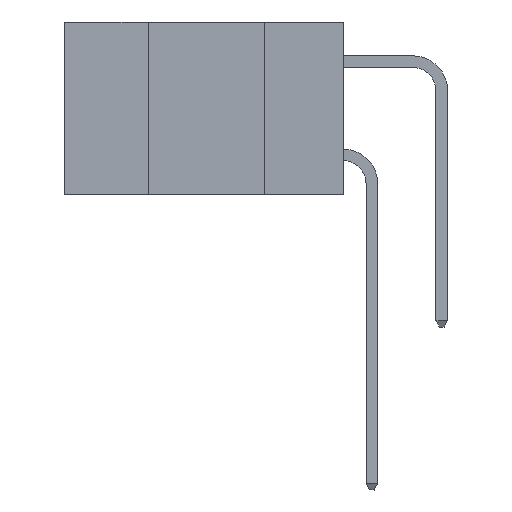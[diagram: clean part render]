
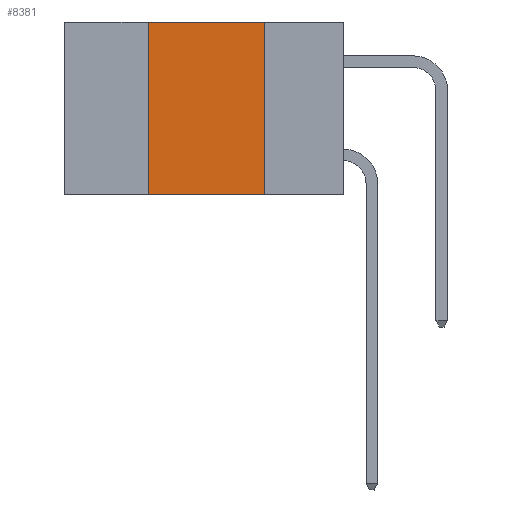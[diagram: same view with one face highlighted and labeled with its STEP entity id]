
A CAD part, left-side view. The second image highlights one B-rep face of the part: STEP entity #8381.
In plain terms, the highlighted planar face has unit normal (-1, 0, 0).
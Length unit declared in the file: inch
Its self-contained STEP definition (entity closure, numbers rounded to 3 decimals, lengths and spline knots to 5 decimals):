
#373 = VERTEX_POINT ( 'NONE', #10980 ) ;
#387 = LINE ( 'NONE', #440, #10869 ) ;
#440 = CARTESIAN_POINT ( 'NONE',  ( 0., 0.6, -0.37 ) ) ;
#542 = CARTESIAN_POINT ( 'NONE',  ( 0., 0.42, -0.37 ) ) ;
#835 = CARTESIAN_POINT ( 'NONE',  ( 0., 0.6, 0. ) ) ;
#958 = ORIENTED_EDGE ( 'NONE', *, *, #9473, .F. ) ;
#2088 = EDGE_CURVE ( 'NONE', #373, #5989, #387, .T. ) ;
#2133 = ORIENTED_EDGE ( 'NONE', *, *, #7985, .F. ) ;
#2447 = EDGE_CURVE ( 'NONE', #2599, #5989, #9921, .T. ) ;
#2492 = VECTOR ( 'NONE', #5140, 39.37008 ) ;
#2599 = VERTEX_POINT ( 'NONE', #11476 ) ;
#3918 = DIRECTION ( 'NONE',  ( 0., 0., -1. ) ) ;
#3961 = LINE ( 'NONE', #9035, #8704 ) ;
#5140 = DIRECTION ( 'NONE',  ( 0., 0., 1. ) ) ;
#5313 = VECTOR ( 'NONE', #3918, 39.37008 ) ;
#5989 = VERTEX_POINT ( 'NONE', #7119 ) ;
#6119 = FACE_OUTER_BOUND ( 'NONE', #9298, .T. ) ;
#7119 = CARTESIAN_POINT ( 'NONE',  ( 0., 0.17, -0.37 ) ) ;
#7619 = CARTESIAN_POINT ( 'NONE',  ( 0., 0.42, 0. ) ) ;
#7925 = DIRECTION ( 'NONE',  ( 1., 0., 0. ) ) ;
#7970 = AXIS2_PLACEMENT_3D ( 'NONE', #835, #7925, #11471 ) ;
#7985 = EDGE_CURVE ( 'NONE', #11083, #2599, #3961, .T. ) ;
#8311 = ORIENTED_EDGE ( 'NONE', *, *, #2447, .F. ) ;
#8381 = ADVANCED_FACE ( 'NONE', ( #6119 ), #9680, .F. ) ;
#8430 = LINE ( 'NONE', #542, #2492 ) ;
#8704 = VECTOR ( 'NONE', #9205, 39.37008 ) ;
#9035 = CARTESIAN_POINT ( 'NONE',  ( 0., 0.6, 0. ) ) ;
#9205 = DIRECTION ( 'NONE',  ( 0., -1., 0. ) ) ;
#9298 = EDGE_LOOP ( 'NONE', ( #8311, #2133, #958, #11392 ) ) ;
#9473 = EDGE_CURVE ( 'NONE', #373, #11083, #8430, .T. ) ;
#9680 = PLANE ( 'NONE',  #7970 ) ;
#9921 = LINE ( 'NONE', #10095, #5313 ) ;
#10095 = CARTESIAN_POINT ( 'NONE',  ( 0., 0.17, -0.37 ) ) ;
#10861 = DIRECTION ( 'NONE',  ( 0., -1., 0. ) ) ;
#10869 = VECTOR ( 'NONE', #10861, 39.37008 ) ;
#10980 = CARTESIAN_POINT ( 'NONE',  ( 0., 0.42, -0.37 ) ) ;
#11083 = VERTEX_POINT ( 'NONE', #7619 ) ;
#11392 = ORIENTED_EDGE ( 'NONE', *, *, #2088, .T. ) ;
#11471 = DIRECTION ( 'NONE',  ( 0., 0., -1. ) ) ;
#11476 = CARTESIAN_POINT ( 'NONE',  ( 0., 0.17, 0. ) ) ;
